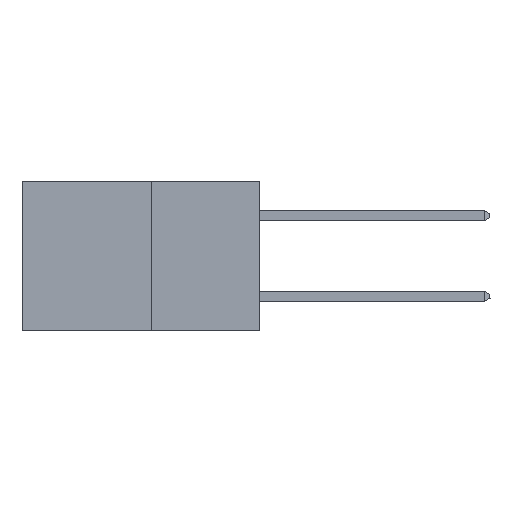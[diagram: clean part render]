
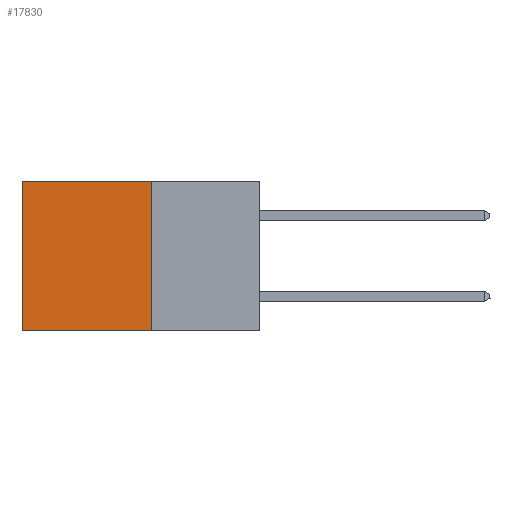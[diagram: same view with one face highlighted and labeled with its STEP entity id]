
A CAD part, left-side view. The second image highlights one B-rep face of the part: STEP entity #17830.
In plain terms, the highlighted planar face has unit normal (-1, 0, 0).
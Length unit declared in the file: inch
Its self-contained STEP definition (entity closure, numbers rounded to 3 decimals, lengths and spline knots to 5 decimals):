
#1519 = CARTESIAN_POINT ( 'NONE',  ( 0.277, 0.27, 0. ) ) ;
#1533 = VERTEX_POINT ( 'NONE', #14677 ) ;
#1736 = DIRECTION ( 'NONE',  ( 0., 0., -1. ) ) ;
#2079 = ORIENTED_EDGE ( 'NONE', *, *, #7747, .F. ) ;
#3018 = FACE_OUTER_BOUND ( 'NONE', #11453, .T. ) ;
#4644 = DIRECTION ( 'NONE',  ( 0., 0., -1. ) ) ;
#5576 = EDGE_CURVE ( 'NONE', #1533, #24484, #17280, .T. ) ;
#6431 = LINE ( 'NONE', #16795, #16530 ) ;
#6670 = LINE ( 'NONE', #8464, #16164 ) ;
#7747 = EDGE_CURVE ( 'NONE', #9504, #24484, #19902, .T. ) ;
#8464 = CARTESIAN_POINT ( 'NONE',  ( 0.277, 0.27, 0. ) ) ;
#9504 = VERTEX_POINT ( 'NONE', #17245 ) ;
#9898 = CARTESIAN_POINT ( 'NONE',  ( 0.277, 0.59, -0.37 ) ) ;
#10393 = DIRECTION ( 'NONE',  ( 0., 1., 0. ) ) ;
#11218 = CARTESIAN_POINT ( 'NONE',  ( 0.277, 0.59, -0.37 ) ) ;
#11453 = EDGE_LOOP ( 'NONE', ( #11524, #2079, #14810, #17771 ) ) ;
#11524 = ORIENTED_EDGE ( 'NONE', *, *, #5576, .T. ) ;
#12124 = DIRECTION ( 'NONE',  ( 0., 1., 0. ) ) ;
#12950 = AXIS2_PLACEMENT_3D ( 'NONE', #19727, #16025, #4644 ) ;
#13983 = CARTESIAN_POINT ( 'NONE',  ( 0.277, 0.27, -0.37 ) ) ;
#14066 = PLANE ( 'NONE',  #12950 ) ;
#14677 = CARTESIAN_POINT ( 'NONE',  ( 0.277, 0.59, 0. ) ) ;
#14810 = ORIENTED_EDGE ( 'NONE', *, *, #20875, .F. ) ;
#14890 = DIRECTION ( 'NONE',  ( 0., 0., -1. ) ) ;
#15671 = VERTEX_POINT ( 'NONE', #1519 ) ;
#16025 = DIRECTION ( 'NONE',  ( 1., 0., 0. ) ) ;
#16164 = VECTOR ( 'NONE', #10393, 39.37008 ) ;
#16530 = VECTOR ( 'NONE', #14890, 39.37008 ) ;
#16795 = CARTESIAN_POINT ( 'NONE',  ( 0.277, 0.27, -0.37 ) ) ;
#17245 = CARTESIAN_POINT ( 'NONE',  ( 0.277, 0.27, -0.37 ) ) ;
#17280 = LINE ( 'NONE', #11218, #21728 ) ;
#17771 = ORIENTED_EDGE ( 'NONE', *, *, #21970, .T. ) ;
#17830 = ADVANCED_FACE ( 'NONE', ( #3018 ), #14066, .F. ) ;
#19294 = VECTOR ( 'NONE', #12124, 39.37008 ) ;
#19727 = CARTESIAN_POINT ( 'NONE',  ( 0.277, 0.27, -0.37 ) ) ;
#19902 = LINE ( 'NONE', #13983, #19294 ) ;
#20875 = EDGE_CURVE ( 'NONE', #15671, #9504, #6431, .T. ) ;
#21728 = VECTOR ( 'NONE', #1736, 39.37008 ) ;
#21970 = EDGE_CURVE ( 'NONE', #15671, #1533, #6670, .T. ) ;
#24484 = VERTEX_POINT ( 'NONE', #9898 ) ;
